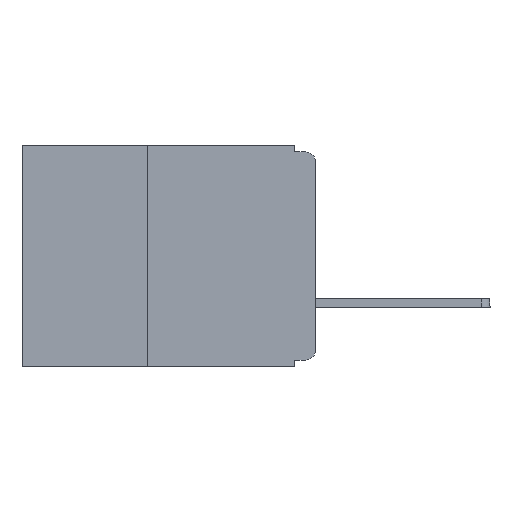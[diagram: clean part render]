
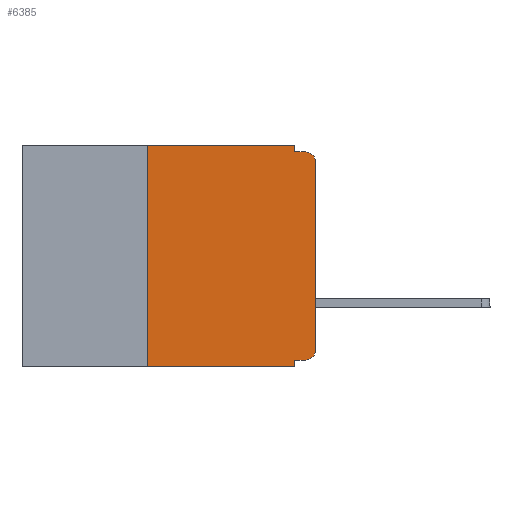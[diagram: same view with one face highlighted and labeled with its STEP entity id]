
A CAD part, left-side view. The second image highlights one B-rep face of the part: STEP entity #6385.
In plain terms, the highlighted planar face has unit normal (-1, 0, 0).
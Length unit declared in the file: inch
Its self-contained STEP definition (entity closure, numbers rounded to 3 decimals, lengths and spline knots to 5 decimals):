
#795 = DIRECTION ( 'NONE',  ( 0., 0., -1. ) ) ;
#803 = DIRECTION ( 'NONE',  ( 0., -1., 0. ) ) ;
#1069 = DIRECTION ( 'NONE',  ( 0., 0., -1. ) ) ;
#1385 = LINE ( 'NONE', #27749, #15246 ) ;
#2074 = ORIENTED_EDGE ( 'NONE', *, *, #17005, .F. ) ;
#2149 = CIRCLE ( 'NONE', #17834, 0.015 ) ;
#2954 = CARTESIAN_POINT ( 'NONE',  ( 0., 0.031, 0. ) ) ;
#3377 = LINE ( 'NONE', #4095, #20659 ) ;
#3521 = DIRECTION ( 'NONE',  ( 0., 0., 1. ) ) ;
#4092 = VECTOR ( 'NONE', #803, 39.37008 ) ;
#4095 = CARTESIAN_POINT ( 'NONE',  ( 0., 0., -0.32 ) ) ;
#4165 = ORIENTED_EDGE ( 'NONE', *, *, #29316, .F. ) ;
#4563 = VECTOR ( 'NONE', #3521, 39.37008 ) ;
#5592 = CARTESIAN_POINT ( 'NONE',  ( 0., 0.437, -0.33 ) ) ;
#6319 = LINE ( 'NONE', #5592, #19386 ) ;
#6345 = AXIS2_PLACEMENT_3D ( 'NONE', #6976, #6763, #6549 ) ;
#6385 = ADVANCED_FACE ( 'NONE', ( #21998 ), #6938, .F. ) ;
#6549 = DIRECTION ( 'NONE',  ( 0., 0., -1. ) ) ;
#6763 = DIRECTION ( 'NONE',  ( 1., 0., 0. ) ) ;
#6808 = ORIENTED_EDGE ( 'NONE', *, *, #29987, .F. ) ;
#6849 = CARTESIAN_POINT ( 'NONE',  ( 0., 0.015, -0.025 ) ) ;
#6938 = PLANE ( 'NONE',  #6345 ) ;
#6976 = CARTESIAN_POINT ( 'NONE',  ( 0., 0.437, 0. ) ) ;
#7714 = CIRCLE ( 'NONE', #21353, 0.015 ) ;
#8224 = VERTEX_POINT ( 'NONE', #19111 ) ;
#9340 = DIRECTION ( 'NONE',  ( 0., 0., -1. ) ) ;
#9965 = VERTEX_POINT ( 'NONE', #28530 ) ;
#10102 = VERTEX_POINT ( 'NONE', #26613 ) ;
#10441 = CARTESIAN_POINT ( 'NONE',  ( 0., 0.015, -0.305 ) ) ;
#10629 = CARTESIAN_POINT ( 'NONE',  ( 0., 0.437, 0. ) ) ;
#11972 = VERTEX_POINT ( 'NONE', #23184 ) ;
#12187 = CARTESIAN_POINT ( 'NONE',  ( 0., 0., 0. ) ) ;
#12878 = VERTEX_POINT ( 'NONE', #27087 ) ;
#12902 = DIRECTION ( 'NONE',  ( 0., 0., -1. ) ) ;
#13076 = ORIENTED_EDGE ( 'NONE', *, *, #14022, .F. ) ;
#13098 = DIRECTION ( 'NONE',  ( 0., -1., 0. ) ) ;
#13299 = CARTESIAN_POINT ( 'NONE',  ( 0., 0.25, -0.33 ) ) ;
#13441 = EDGE_LOOP ( 'NONE', ( #30307, #15567, #2074, #6808, #13076, #29346, #26135, #4165, #19953, #17061 ) ) ;
#14022 = EDGE_CURVE ( 'NONE', #17609, #17586, #18457, .T. ) ;
#14636 = DIRECTION ( 'NONE',  ( 0., 0., 1. ) ) ;
#15246 = VECTOR ( 'NONE', #795, 39.37008 ) ;
#15567 = ORIENTED_EDGE ( 'NONE', *, *, #20798, .T. ) ;
#15929 = EDGE_CURVE ( 'NONE', #12878, #17609, #26783, .T. ) ;
#16337 = DIRECTION ( 'NONE',  ( 0., 1., 0. ) ) ;
#16899 = VECTOR ( 'NONE', #13098, 39.37008 ) ;
#17005 = EDGE_CURVE ( 'NONE', #19572, #11972, #17156, .T. ) ;
#17061 = ORIENTED_EDGE ( 'NONE', *, *, #28642, .T. ) ;
#17156 = LINE ( 'NONE', #18030, #4092 ) ;
#17586 = VERTEX_POINT ( 'NONE', #2954 ) ;
#17609 = VERTEX_POINT ( 'NONE', #22711 ) ;
#17834 = AXIS2_PLACEMENT_3D ( 'NONE', #10441, #27569, #12902 ) ;
#18030 = CARTESIAN_POINT ( 'NONE',  ( 0., 0., -0.01 ) ) ;
#18058 = EDGE_CURVE ( 'NONE', #22793, #18588, #19010, .T. ) ;
#18246 = EDGE_CURVE ( 'NONE', #12878, #9965, #6319, .T. ) ;
#18457 = LINE ( 'NONE', #10629, #16899 ) ;
#18588 = VERTEX_POINT ( 'NONE', #26496 ) ;
#19010 = LINE ( 'NONE', #12187, #31176 ) ;
#19111 = CARTESIAN_POINT ( 'NONE',  ( 0., 0.031, -0.32 ) ) ;
#19158 = CARTESIAN_POINT ( 'NONE',  ( 0., 0.031, -0.01 ) ) ;
#19386 = VECTOR ( 'NONE', #22781, 39.37008 ) ;
#19572 = VERTEX_POINT ( 'NONE', #19158 ) ;
#19953 = ORIENTED_EDGE ( 'NONE', *, *, #24410, .F. ) ;
#20659 = VECTOR ( 'NONE', #16337, 39.37008 ) ;
#20798 = EDGE_CURVE ( 'NONE', #18588, #11972, #7714, .T. ) ;
#21353 = AXIS2_PLACEMENT_3D ( 'NONE', #6849, #24023, #9340 ) ;
#21998 = FACE_OUTER_BOUND ( 'NONE', #13441, .T. ) ;
#22711 = CARTESIAN_POINT ( 'NONE',  ( 0., 0.25, 0. ) ) ;
#22781 = DIRECTION ( 'NONE',  ( 0., -1., 0. ) ) ;
#22793 = VERTEX_POINT ( 'NONE', #29581 ) ;
#23184 = CARTESIAN_POINT ( 'NONE',  ( 0., 0.015, -0.01 ) ) ;
#24023 = DIRECTION ( 'NONE',  ( -1., 0., 0. ) ) ;
#24410 = EDGE_CURVE ( 'NONE', #10102, #8224, #3377, .T. ) ;
#25570 = VECTOR ( 'NONE', #1069, 39.37008 ) ;
#26135 = ORIENTED_EDGE ( 'NONE', *, *, #18246, .T. ) ;
#26319 = LINE ( 'NONE', #28028, #25570 ) ;
#26496 = CARTESIAN_POINT ( 'NONE',  ( 0., 0., -0.025 ) ) ;
#26613 = CARTESIAN_POINT ( 'NONE',  ( 0., 0.015, -0.32 ) ) ;
#26783 = LINE ( 'NONE', #13299, #4563 ) ;
#27087 = CARTESIAN_POINT ( 'NONE',  ( 0., 0.25, -0.33 ) ) ;
#27569 = DIRECTION ( 'NONE',  ( -1., 0., 0. ) ) ;
#27749 = CARTESIAN_POINT ( 'NONE',  ( 0., 0.031, -0.33 ) ) ;
#28028 = CARTESIAN_POINT ( 'NONE',  ( 0., 0.031, 0. ) ) ;
#28530 = CARTESIAN_POINT ( 'NONE',  ( 0., 0.031, -0.33 ) ) ;
#28642 = EDGE_CURVE ( 'NONE', #10102, #22793, #2149, .T. ) ;
#29316 = EDGE_CURVE ( 'NONE', #8224, #9965, #1385, .T. ) ;
#29346 = ORIENTED_EDGE ( 'NONE', *, *, #15929, .F. ) ;
#29581 = CARTESIAN_POINT ( 'NONE',  ( 0., 0., -0.305 ) ) ;
#29987 = EDGE_CURVE ( 'NONE', #17586, #19572, #26319, .T. ) ;
#30307 = ORIENTED_EDGE ( 'NONE', *, *, #18058, .T. ) ;
#31176 = VECTOR ( 'NONE', #14636, 39.37008 ) ;
